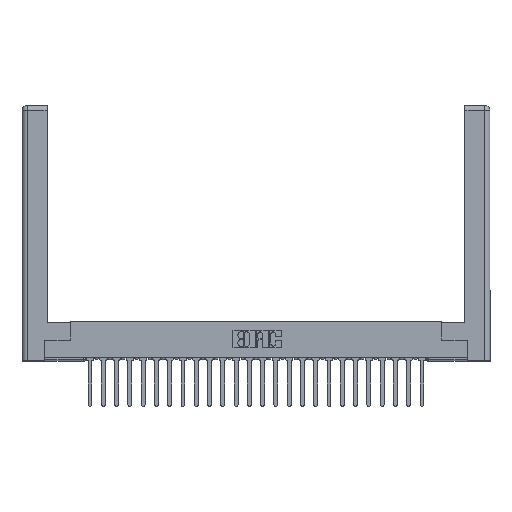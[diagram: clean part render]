
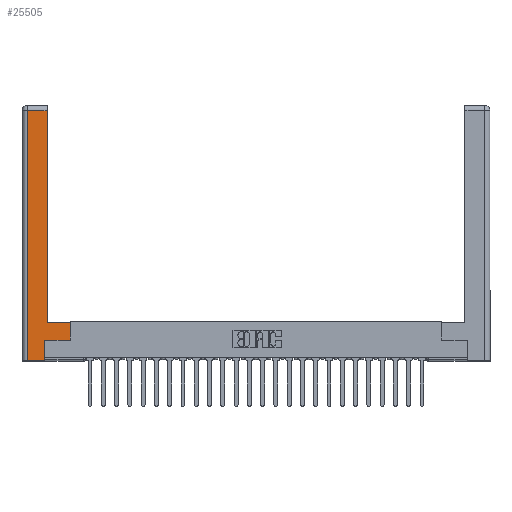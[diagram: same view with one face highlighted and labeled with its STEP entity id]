
A CAD part, top view. The second image highlights one B-rep face of the part: STEP entity #25505.
In plain terms, the highlighted planar face has unit normal (0, 0, 1).
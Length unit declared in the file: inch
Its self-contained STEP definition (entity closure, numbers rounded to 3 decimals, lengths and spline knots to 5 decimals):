
#109 = DIRECTION ( 'NONE',  ( 0., 0., -1. ) ) ;
#202 = CARTESIAN_POINT ( 'NONE',  ( 0.265, 0.245, 0. ) ) ;
#536 = CARTESIAN_POINT ( 'NONE',  ( 0., 0., 0. ) ) ;
#1058 = LINE ( 'NONE', #18580, #18929 ) ;
#1747 = DIRECTION ( 'NONE',  ( -1., 0., 0. ) ) ;
#1787 = DIRECTION ( 'NONE',  ( 0., 1., 0. ) ) ;
#1989 = VECTOR ( 'NONE', #18884, 39.37008 ) ;
#2061 = CARTESIAN_POINT ( 'NONE',  ( 0.0615, 0., 0. ) ) ;
#2378 = DIRECTION ( 'NONE',  ( 1., 0., 0. ) ) ;
#2417 = EDGE_CURVE ( 'NONE', #12691, #20829, #19151, .T. ) ;
#2953 = VECTOR ( 'NONE', #1747, 39.37008 ) ;
#4403 = DIRECTION ( 'NONE',  ( 0., 1., 0. ) ) ;
#5450 = ORIENTED_EDGE ( 'NONE', *, *, #17609, .T. ) ;
#5632 = DIRECTION ( 'NONE',  ( -1., 0., 0. ) ) ;
#5941 = ORIENTED_EDGE ( 'NONE', *, *, #15814, .T. ) ;
#6571 = VECTOR ( 'NONE', #8760, 39.37008 ) ;
#7959 = ORIENTED_EDGE ( 'NONE', *, *, #14950, .T. ) ;
#8214 = ORIENTED_EDGE ( 'NONE', *, *, #14824, .T. ) ;
#8760 = DIRECTION ( 'NONE',  ( 0., 1., 0. ) ) ;
#8815 = CARTESIAN_POINT ( 'NONE',  ( 0.265, 0.245, 0. ) ) ;
#9617 = DIRECTION ( 'NONE',  ( 1., 0., 0. ) ) ;
#10920 = ORIENTED_EDGE ( 'NONE', *, *, #2417, .T. ) ;
#12691 = VERTEX_POINT ( 'NONE', #22121 ) ;
#13236 = CARTESIAN_POINT ( 'NONE',  ( 0.0615, 0., 0. ) ) ;
#13377 = LINE ( 'NONE', #24167, #25284 ) ;
#13457 = EDGE_LOOP ( 'NONE', ( #10920, #8214, #5941, #25183, #15765, #15597, #5450, #7959 ) ) ;
#13537 = VERTEX_POINT ( 'NONE', #13236 ) ;
#13680 = FACE_OUTER_BOUND ( 'NONE', #13457, .T. ) ;
#14223 = CARTESIAN_POINT ( 'NONE',  ( 0.295, 0.45, 0. ) ) ;
#14689 = CARTESIAN_POINT ( 'NONE',  ( 0.295, 2.94, 0. ) ) ;
#14824 = EDGE_CURVE ( 'NONE', #20829, #19487, #20760, .T. ) ;
#14950 = EDGE_CURVE ( 'NONE', #15335, #12691, #16459, .T. ) ;
#15335 = VERTEX_POINT ( 'NONE', #17088 ) ;
#15476 = VERTEX_POINT ( 'NONE', #8815 ) ;
#15597 = ORIENTED_EDGE ( 'NONE', *, *, #27543, .T. ) ;
#15765 = ORIENTED_EDGE ( 'NONE', *, *, #20169, .T. ) ;
#15814 = EDGE_CURVE ( 'NONE', #19487, #13537, #27450, .T. ) ;
#16459 = LINE ( 'NONE', #14223, #2953 ) ;
#16525 = VECTOR ( 'NONE', #2378, 39.37008 ) ;
#16976 = CARTESIAN_POINT ( 'NONE',  ( 0.0615, 2.94, 0. ) ) ;
#17088 = CARTESIAN_POINT ( 'NONE',  ( 0.565, 0.45, 0. ) ) ;
#17609 = EDGE_CURVE ( 'NONE', #26348, #15335, #13377, .T. ) ;
#18580 = CARTESIAN_POINT ( 'NONE',  ( 0.565, 0.245, 0. ) ) ;
#18881 = CARTESIAN_POINT ( 'NONE',  ( 0.295, 3., 0. ) ) ;
#18884 = DIRECTION ( 'NONE',  ( 0., -1., 0. ) ) ;
#18929 = VECTOR ( 'NONE', #9617, 39.37008 ) ;
#19151 = LINE ( 'NONE', #18881, #19413 ) ;
#19399 = LINE ( 'NONE', #202, #6571 ) ;
#19413 = VECTOR ( 'NONE', #1787, 39.37008 ) ;
#19487 = VERTEX_POINT ( 'NONE', #22275 ) ;
#19759 = CARTESIAN_POINT ( 'NONE',  ( 0.565, 0.245, 0. ) ) ;
#20169 = EDGE_CURVE ( 'NONE', #26675, #15476, #19399, .T. ) ;
#20181 = AXIS2_PLACEMENT_3D ( 'NONE', #536, #109, #23946 ) ;
#20760 = LINE ( 'NONE', #16976, #24898 ) ;
#20829 = VERTEX_POINT ( 'NONE', #14689 ) ;
#21553 = PLANE ( 'NONE',  #20181 ) ;
#22121 = CARTESIAN_POINT ( 'NONE',  ( 0.295, 0.45, 0. ) ) ;
#22186 = EDGE_CURVE ( 'NONE', #13537, #26675, #23423, .T. ) ;
#22275 = CARTESIAN_POINT ( 'NONE',  ( 0.0615, 2.94, 0. ) ) ;
#23400 = CARTESIAN_POINT ( 'NONE',  ( 0.265, 0., 0. ) ) ;
#23423 = LINE ( 'NONE', #27646, #16525 ) ;
#23946 = DIRECTION ( 'NONE',  ( -1., 0., 0. ) ) ;
#24167 = CARTESIAN_POINT ( 'NONE',  ( 0.565, 0.45, 0. ) ) ;
#24898 = VECTOR ( 'NONE', #5632, 39.37008 ) ;
#25183 = ORIENTED_EDGE ( 'NONE', *, *, #22186, .T. ) ;
#25284 = VECTOR ( 'NONE', #4403, 39.37008 ) ;
#25505 = ADVANCED_FACE ( 'NONE', ( #13680 ), #21553, .F. ) ;
#26348 = VERTEX_POINT ( 'NONE', #19759 ) ;
#26675 = VERTEX_POINT ( 'NONE', #23400 ) ;
#27450 = LINE ( 'NONE', #2061, #1989 ) ;
#27543 = EDGE_CURVE ( 'NONE', #15476, #26348, #1058, .T. ) ;
#27646 = CARTESIAN_POINT ( 'NONE',  ( 0.265, 0., 0. ) ) ;
